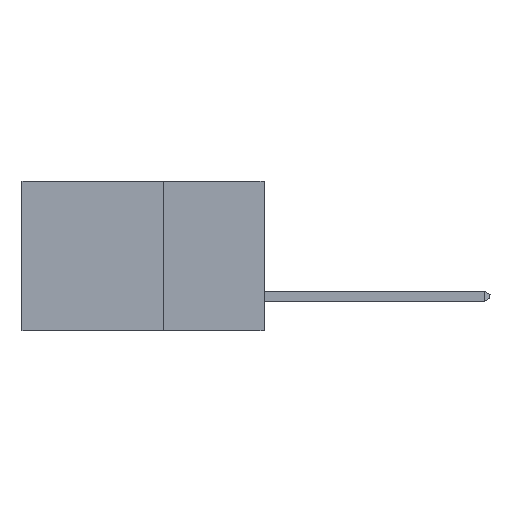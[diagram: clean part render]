
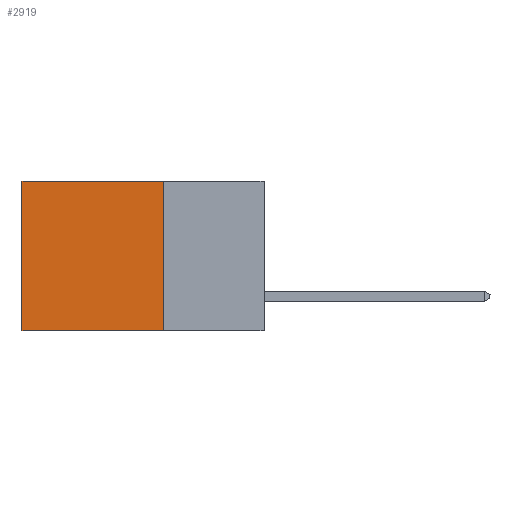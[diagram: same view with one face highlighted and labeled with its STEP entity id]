
A CAD part, left-side view. The second image highlights one B-rep face of the part: STEP entity #2919.
In plain terms, the highlighted planar face has unit normal (-1, 0, 0).
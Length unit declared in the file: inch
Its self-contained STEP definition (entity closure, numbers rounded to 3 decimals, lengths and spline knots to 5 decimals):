
#155 = CARTESIAN_POINT ( 'NONE',  ( 0.298, 0.6, 0. ) ) ;
#396 = CARTESIAN_POINT ( 'NONE',  ( 0.298, 0.25, 0. ) ) ;
#941 = DIRECTION ( 'NONE',  ( 0., 0., -1. ) ) ;
#991 = CARTESIAN_POINT ( 'NONE',  ( 0.298, 0.25, 0. ) ) ;
#1519 = VECTOR ( 'NONE', #8171, 39.37008 ) ;
#2092 = EDGE_CURVE ( 'NONE', #3331, #13645, #6522, .T. ) ;
#2482 = CARTESIAN_POINT ( 'NONE',  ( 0.298, 0.6, -0.37 ) ) ;
#2919 = ADVANCED_FACE ( 'NONE', ( #7484 ), #22127, .F. ) ;
#3331 = VERTEX_POINT ( 'NONE', #155 ) ;
#3953 = DIRECTION ( 'NONE',  ( 0., 1., 0. ) ) ;
#4370 = VECTOR ( 'NONE', #3953, 39.37008 ) ;
#4941 = CARTESIAN_POINT ( 'NONE',  ( 0.298, 0.25, 0. ) ) ;
#5510 = ORIENTED_EDGE ( 'NONE', *, *, #19068, .F. ) ;
#6274 = CARTESIAN_POINT ( 'NONE',  ( 0.298, 0.6, 0. ) ) ;
#6522 = LINE ( 'NONE', #6274, #1519 ) ;
#7484 = FACE_OUTER_BOUND ( 'NONE', #11379, .T. ) ;
#7564 = CARTESIAN_POINT ( 'NONE',  ( 0.298, 0.25, 0. ) ) ;
#7728 = ORIENTED_EDGE ( 'NONE', *, *, #22201, .F. ) ;
#7745 = AXIS2_PLACEMENT_3D ( 'NONE', #991, #18124, #12424 ) ;
#8171 = DIRECTION ( 'NONE',  ( 0., 0., -1. ) ) ;
#8179 = LINE ( 'NONE', #7564, #4370 ) ;
#8740 = CARTESIAN_POINT ( 'NONE',  ( 0.298, 0.25, -0.37 ) ) ;
#11379 = EDGE_LOOP ( 'NONE', ( #15028, #7728, #5510, #21545 ) ) ;
#12424 = DIRECTION ( 'NONE',  ( 0., 0., -1. ) ) ;
#12752 = VECTOR ( 'NONE', #18535, 39.37008 ) ;
#13112 = EDGE_CURVE ( 'NONE', #21506, #3331, #8179, .T. ) ;
#13645 = VERTEX_POINT ( 'NONE', #2482 ) ;
#15028 = ORIENTED_EDGE ( 'NONE', *, *, #2092, .T. ) ;
#16003 = LINE ( 'NONE', #18461, #12752 ) ;
#18124 = DIRECTION ( 'NONE',  ( 1., 0., 0. ) ) ;
#18461 = CARTESIAN_POINT ( 'NONE',  ( 0.298, 0.25, -0.37 ) ) ;
#18535 = DIRECTION ( 'NONE',  ( 0., 1., 0. ) ) ;
#19068 = EDGE_CURVE ( 'NONE', #21506, #22694, #20777, .T. ) ;
#19922 = VECTOR ( 'NONE', #941, 39.37008 ) ;
#20777 = LINE ( 'NONE', #4941, #19922 ) ;
#21506 = VERTEX_POINT ( 'NONE', #396 ) ;
#21545 = ORIENTED_EDGE ( 'NONE', *, *, #13112, .T. ) ;
#22127 = PLANE ( 'NONE',  #7745 ) ;
#22201 = EDGE_CURVE ( 'NONE', #22694, #13645, #16003, .T. ) ;
#22694 = VERTEX_POINT ( 'NONE', #8740 ) ;
